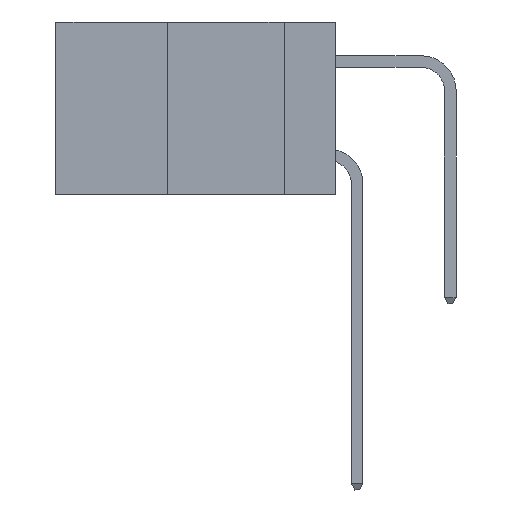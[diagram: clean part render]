
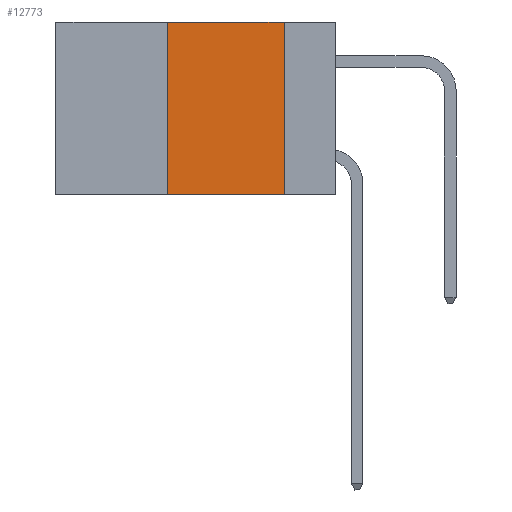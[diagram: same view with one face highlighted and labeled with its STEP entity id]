
A CAD part, left-side view. The second image highlights one B-rep face of the part: STEP entity #12773.
In plain terms, the highlighted planar face has unit normal (-1, 0, 0).
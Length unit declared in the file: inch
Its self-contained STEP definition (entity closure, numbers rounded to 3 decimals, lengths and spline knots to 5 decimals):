
#131 = LINE ( 'NONE', #2417, #3553 ) ;
#593 = LINE ( 'NONE', #2356, #1824 ) ;
#658 = ORIENTED_EDGE ( 'NONE', *, *, #23500, .F. ) ;
#1824 = VECTOR ( 'NONE', #10212, 39.37008 ) ;
#2356 = CARTESIAN_POINT ( 'NONE',  ( 0., 0.6, 0. ) ) ;
#2417 = CARTESIAN_POINT ( 'NONE',  ( 0., 0.36, 0. ) ) ;
#2464 = EDGE_LOOP ( 'NONE', ( #24580, #12283, #658, #12897 ) ) ;
#3336 = LINE ( 'NONE', #6236, #7349 ) ;
#3553 = VECTOR ( 'NONE', #8449, 39.37008 ) ;
#3816 = VERTEX_POINT ( 'NONE', #23168 ) ;
#4398 = DIRECTION ( 'NONE',  ( 0., 0., -1. ) ) ;
#5135 = PLANE ( 'NONE',  #6973 ) ;
#5246 = VERTEX_POINT ( 'NONE', #15852 ) ;
#6236 = CARTESIAN_POINT ( 'NONE',  ( 0., 0.11, 0. ) ) ;
#6894 = EDGE_CURVE ( 'NONE', #3816, #5246, #593, .T. ) ;
#6973 = AXIS2_PLACEMENT_3D ( 'NONE', #20921, #23662, #8059 ) ;
#7349 = VECTOR ( 'NONE', #4398, 39.37008 ) ;
#7730 = EDGE_CURVE ( 'NONE', #5246, #24294, #3336, .T. ) ;
#7751 = CARTESIAN_POINT ( 'NONE',  ( 0., 0.11, -0.37 ) ) ;
#8059 = DIRECTION ( 'NONE',  ( 0., 0., -1. ) ) ;
#8449 = DIRECTION ( 'NONE',  ( 0., 0., 1. ) ) ;
#8934 = DIRECTION ( 'NONE',  ( 0., -1., 0. ) ) ;
#9969 = FACE_OUTER_BOUND ( 'NONE', #2464, .T. ) ;
#10212 = DIRECTION ( 'NONE',  ( 0., -1., 0. ) ) ;
#10914 = CARTESIAN_POINT ( 'NONE',  ( 0., 0.6, -0.37 ) ) ;
#12283 = ORIENTED_EDGE ( 'NONE', *, *, #6894, .F. ) ;
#12773 = ADVANCED_FACE ( 'NONE', ( #9969 ), #5135, .F. ) ;
#12897 = ORIENTED_EDGE ( 'NONE', *, *, #17304, .T. ) ;
#13168 = CARTESIAN_POINT ( 'NONE',  ( 0., 0.36, -0.37 ) ) ;
#13913 = VECTOR ( 'NONE', #8934, 39.37008 ) ;
#15454 = LINE ( 'NONE', #10914, #13913 ) ;
#15852 = CARTESIAN_POINT ( 'NONE',  ( 0., 0.11, 0. ) ) ;
#17304 = EDGE_CURVE ( 'NONE', #17537, #24294, #15454, .T. ) ;
#17537 = VERTEX_POINT ( 'NONE', #13168 ) ;
#20921 = CARTESIAN_POINT ( 'NONE',  ( 0., 0.6, 0. ) ) ;
#23168 = CARTESIAN_POINT ( 'NONE',  ( 0., 0.36, 0. ) ) ;
#23500 = EDGE_CURVE ( 'NONE', #17537, #3816, #131, .T. ) ;
#23662 = DIRECTION ( 'NONE',  ( 1., 0., 0. ) ) ;
#24294 = VERTEX_POINT ( 'NONE', #7751 ) ;
#24580 = ORIENTED_EDGE ( 'NONE', *, *, #7730, .F. ) ;
